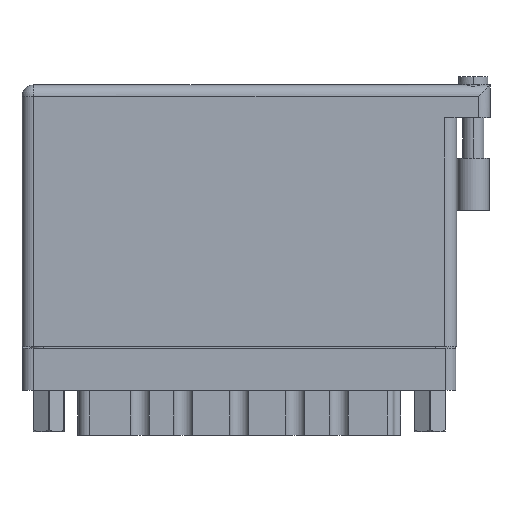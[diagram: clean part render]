
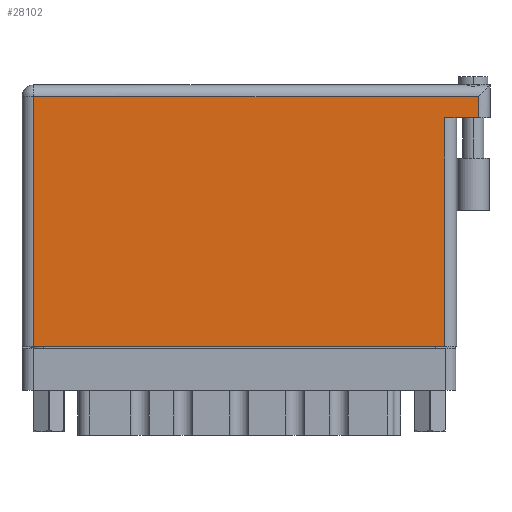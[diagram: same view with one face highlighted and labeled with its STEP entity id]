
A CAD part, front view. The second image highlights one B-rep face of the part: STEP entity #28102.
In plain terms, the highlighted face is planar.
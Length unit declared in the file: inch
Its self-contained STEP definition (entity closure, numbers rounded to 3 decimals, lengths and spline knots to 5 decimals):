
#3048 = DIRECTION ( 'NONE',  ( 0., 0., -1. ) ) ;
#3929 = PLANE ( 'NONE',  #26752 ) ;
#4921 = CARTESIAN_POINT ( 'NONE',  ( 0., 0., 0. ) ) ;
#6072 = VECTOR ( 'NONE', #17318, 39.37008 ) ;
#6540 = CARTESIAN_POINT ( 'NONE',  ( 2.73, 1.566, 0. ) ) ;
#7036 = ORIENTED_EDGE ( 'NONE', *, *, #14601, .T. ) ;
#7621 = CARTESIAN_POINT ( 'NONE',  ( 0., 1.566, 0. ) ) ;
#8403 = ORIENTED_EDGE ( 'NONE', *, *, #11009, .T. ) ;
#11009 = EDGE_CURVE ( 'NONE', #13843, #55731, #35644, .T. ) ;
#11158 = EDGE_CURVE ( 'NONE', #55731, #19174, #12769, .T. ) ;
#12769 = LINE ( 'NONE', #27561, #43210 ) ;
#13843 = VERTEX_POINT ( 'NONE', #54129 ) ;
#14537 = EDGE_LOOP ( 'NONE', ( #8403, #41142, #35118, #7036, #38891, #29005 ) ) ;
#14601 = EDGE_CURVE ( 'NONE', #45161, #31758, #28204, .T. ) ;
#16588 = LINE ( 'NONE', #35689, #25478 ) ;
#16920 = VECTOR ( 'NONE', #44847, 39.37008 ) ;
#17318 = DIRECTION ( 'NONE',  ( 0., -1., 0. ) ) ;
#17826 = VECTOR ( 'NONE', #19499, 39.37008 ) ;
#19174 = VERTEX_POINT ( 'NONE', #44965 ) ;
#19499 = DIRECTION ( 'NONE',  ( 0., 1., 0. ) ) ;
#20082 = DIRECTION ( 'NONE',  ( -1., 0., 0. ) ) ;
#20266 = EDGE_CURVE ( 'NONE', #56188, #13843, #37940, .T. ) ;
#20771 = DIRECTION ( 'NONE',  ( -1., 0., 0. ) ) ;
#22575 = LINE ( 'NONE', #36720, #37888 ) ;
#23892 = DIRECTION ( 'NONE',  ( -1., 0., 0. ) ) ;
#25478 = VECTOR ( 'NONE', #20771, 39.37008 ) ;
#26752 = AXIS2_PLACEMENT_3D ( 'NONE', #7621, #3048, #20082 ) ;
#27561 = CARTESIAN_POINT ( 'NONE',  ( 2.53, 1.369, 0. ) ) ;
#28102 = ADVANCED_FACE ( 'NONE', ( #41566 ), #3929, .F. ) ;
#28204 = LINE ( 'NONE', #6540, #17826 ) ;
#29005 = ORIENTED_EDGE ( 'NONE', *, *, #20266, .T. ) ;
#31758 = VERTEX_POINT ( 'NONE', #49718 ) ;
#32045 = EDGE_CURVE ( 'NONE', #31758, #56188, #16588, .T. ) ;
#35118 = ORIENTED_EDGE ( 'NONE', *, *, #43833, .F. ) ;
#35644 = LINE ( 'NONE', #4921, #16920 ) ;
#35689 = CARTESIAN_POINT ( 'NONE',  ( 0., 1.496, 0. ) ) ;
#36720 = CARTESIAN_POINT ( 'NONE',  ( 2.8, 1.369, 0. ) ) ;
#37888 = VECTOR ( 'NONE', #23892, 39.37008 ) ;
#37940 = LINE ( 'NONE', #44245, #6072 ) ;
#38891 = ORIENTED_EDGE ( 'NONE', *, *, #32045, .T. ) ;
#40950 = DIRECTION ( 'NONE',  ( 0., 1., 0. ) ) ;
#41142 = ORIENTED_EDGE ( 'NONE', *, *, #11158, .T. ) ;
#41566 = FACE_OUTER_BOUND ( 'NONE', #14537, .T. ) ;
#43210 = VECTOR ( 'NONE', #40950, 39.37008 ) ;
#43833 = EDGE_CURVE ( 'NONE', #45161, #19174, #22575, .T. ) ;
#44245 = CARTESIAN_POINT ( 'NONE',  ( 0.07, 0., 0. ) ) ;
#44847 = DIRECTION ( 'NONE',  ( 1., 0., 0. ) ) ;
#44965 = CARTESIAN_POINT ( 'NONE',  ( 2.53, 1.369, 0. ) ) ;
#45161 = VERTEX_POINT ( 'NONE', #50370 ) ;
#49718 = CARTESIAN_POINT ( 'NONE',  ( 2.73, 1.496, 0. ) ) ;
#50370 = CARTESIAN_POINT ( 'NONE',  ( 2.73, 1.369, 0. ) ) ;
#52801 = CARTESIAN_POINT ( 'NONE',  ( 2.53, 0., 0. ) ) ;
#54129 = CARTESIAN_POINT ( 'NONE',  ( 0.07, 0., 0. ) ) ;
#55020 = CARTESIAN_POINT ( 'NONE',  ( 0.07, 1.496, 0. ) ) ;
#55731 = VERTEX_POINT ( 'NONE', #52801 ) ;
#56188 = VERTEX_POINT ( 'NONE', #55020 ) ;
